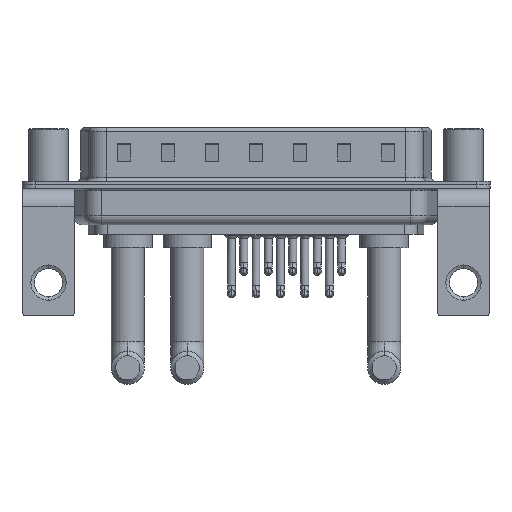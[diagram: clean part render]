
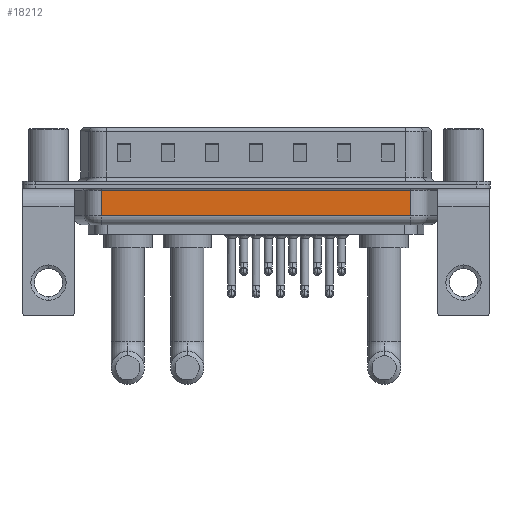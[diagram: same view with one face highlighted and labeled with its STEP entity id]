
A CAD part, front view. The second image highlights one B-rep face of the part: STEP entity #18212.
In plain terms, the highlighted planar face has unit normal (0, -1, 0).
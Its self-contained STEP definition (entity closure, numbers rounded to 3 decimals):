
#229 = VERTEX_POINT ( 'NONE', #7681 ) ;
#466 = CARTESIAN_POINT ( 'NONE',  ( 41.044, -5.35, -4.5 ) ) ;
#2724 = DIRECTION ( 'NONE',  ( 0., 0., 1. ) ) ;
#3595 = VECTOR ( 'NONE', #2724, 1000. ) ;
#4108 = CARTESIAN_POINT ( 'NONE',  ( 6.006, -5.35, -0.65 ) ) ;
#4182 = CARTESIAN_POINT ( 'NONE',  ( 6.006, -5.35, -3.5 ) ) ;
#4471 = VECTOR ( 'NONE', #15609, 1000. ) ;
#4952 = EDGE_LOOP ( 'NONE', ( #21482, #14102, #12145, #13089 ) ) ;
#5207 = PLANE ( 'NONE',  #16121 ) ;
#5530 = EDGE_CURVE ( 'NONE', #13615, #229, #19687, .T. ) ;
#6661 = EDGE_CURVE ( 'NONE', #22325, #14482, #10615, .T. ) ;
#7075 = VECTOR ( 'NONE', #16711, 1000. ) ;
#7681 = CARTESIAN_POINT ( 'NONE',  ( 41.044, -5.35, -3.5 ) ) ;
#9524 = LINE ( 'NONE', #17594, #4471 ) ;
#10615 = LINE ( 'NONE', #14576, #7075 ) ;
#12145 = ORIENTED_EDGE ( 'NONE', *, *, #22763, .T. ) ;
#13089 = ORIENTED_EDGE ( 'NONE', *, *, #6661, .T. ) ;
#13615 = VERTEX_POINT ( 'NONE', #4182 ) ;
#14102 = ORIENTED_EDGE ( 'NONE', *, *, #5530, .T. ) ;
#14482 = VERTEX_POINT ( 'NONE', #4108 ) ;
#14576 = CARTESIAN_POINT ( 'NONE',  ( 6.006, -5.35, -0.65 ) ) ;
#15609 = DIRECTION ( 'NONE',  ( 0., 0., 1. ) ) ;
#15615 = CARTESIAN_POINT ( 'NONE',  ( 6.006, -5.35, -4.5 ) ) ;
#15743 = FACE_OUTER_BOUND ( 'NONE', #4952, .T. ) ;
#16121 = AXIS2_PLACEMENT_3D ( 'NONE', #15615, #17469, #25258 ) ;
#16711 = DIRECTION ( 'NONE',  ( -1., 0., 0. ) ) ;
#17469 = DIRECTION ( 'NONE',  ( 0., 1., 0. ) ) ;
#17594 = CARTESIAN_POINT ( 'NONE',  ( 6.006, -5.35, -4.5 ) ) ;
#18212 = ADVANCED_FACE ( 'NONE', ( #15743 ), #5207, .F. ) ;
#19435 = CARTESIAN_POINT ( 'NONE',  ( 6.006, -5.35, -3.5 ) ) ;
#19687 = LINE ( 'NONE', #19435, #25550 ) ;
#21190 = LINE ( 'NONE', #466, #3595 ) ;
#21482 = ORIENTED_EDGE ( 'NONE', *, *, #23384, .F. ) ;
#22325 = VERTEX_POINT ( 'NONE', #22668 ) ;
#22668 = CARTESIAN_POINT ( 'NONE',  ( 41.044, -5.35, -0.65 ) ) ;
#22763 = EDGE_CURVE ( 'NONE', #229, #22325, #21190, .T. ) ;
#23384 = EDGE_CURVE ( 'NONE', #13615, #14482, #9524, .T. ) ;
#25258 = DIRECTION ( 'NONE',  ( 0., 0., 1. ) ) ;
#25550 = VECTOR ( 'NONE', #25630, 1000. ) ;
#25630 = DIRECTION ( 'NONE',  ( 1., 0., 0. ) ) ;
